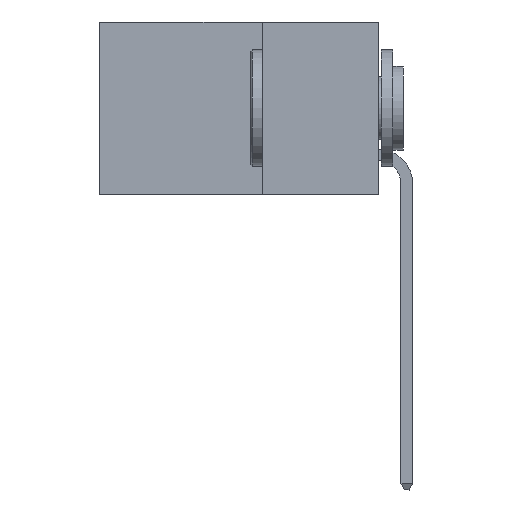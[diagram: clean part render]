
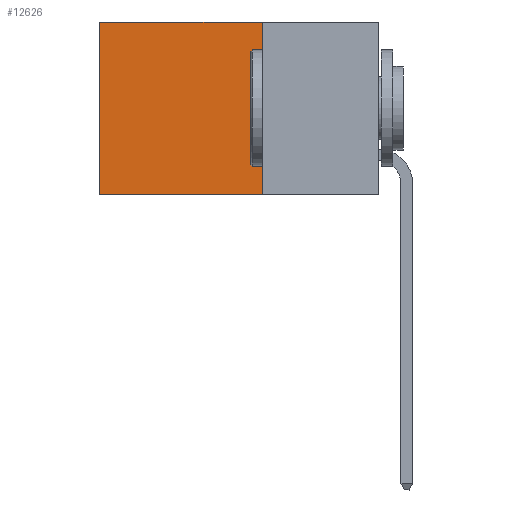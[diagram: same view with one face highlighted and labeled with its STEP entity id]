
A CAD part, left-side view. The second image highlights one B-rep face of the part: STEP entity #12626.
In plain terms, the highlighted planar face has unit normal (-1, 0, 0).
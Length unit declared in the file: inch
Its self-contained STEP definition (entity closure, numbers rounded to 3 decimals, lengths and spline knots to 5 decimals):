
#63 = CARTESIAN_POINT ( 'NONE',  ( 0.298, 0.25, -0.37 ) ) ;
#999 = PLANE ( 'NONE',  #11943 ) ;
#2259 = DIRECTION ( 'NONE',  ( 0., 0., -1. ) ) ;
#3012 = FACE_OUTER_BOUND ( 'NONE', #7542, .T. ) ;
#3633 = CARTESIAN_POINT ( 'NONE',  ( 0.298, 0.6, 0. ) ) ;
#3828 = DIRECTION ( 'NONE',  ( 0., 0., -1. ) ) ;
#4399 = VECTOR ( 'NONE', #9729, 39.37008 ) ;
#5087 = VECTOR ( 'NONE', #11997, 39.37008 ) ;
#5766 = VECTOR ( 'NONE', #6267, 39.37008 ) ;
#6267 = DIRECTION ( 'NONE',  ( 0., 1., 0. ) ) ;
#7542 = EDGE_LOOP ( 'NONE', ( #9388, #9931, #10273, #8222 ) ) ;
#7642 = VECTOR ( 'NONE', #3828, 39.37008 ) ;
#8222 = ORIENTED_EDGE ( 'NONE', *, *, #15827, .T. ) ;
#9388 = ORIENTED_EDGE ( 'NONE', *, *, #12764, .T. ) ;
#9648 = DIRECTION ( 'NONE',  ( 1., 0., 0. ) ) ;
#9729 = DIRECTION ( 'NONE',  ( 0., 0., -1. ) ) ;
#9931 = ORIENTED_EDGE ( 'NONE', *, *, #10472, .F. ) ;
#10273 = ORIENTED_EDGE ( 'NONE', *, *, #10363, .F. ) ;
#10280 = CARTESIAN_POINT ( 'NONE',  ( 0.298, 0.25, 0. ) ) ;
#10363 = EDGE_CURVE ( 'NONE', #15689, #11146, #13837, .T. ) ;
#10472 = EDGE_CURVE ( 'NONE', #11146, #15243, #15586, .T. ) ;
#10766 = CARTESIAN_POINT ( 'NONE',  ( 0.298, 0.25, 0. ) ) ;
#11146 = VERTEX_POINT ( 'NONE', #14893 ) ;
#11212 = CARTESIAN_POINT ( 'NONE',  ( 0.298, 0.6, 0. ) ) ;
#11943 = AXIS2_PLACEMENT_3D ( 'NONE', #15807, #9648, #2259 ) ;
#11997 = DIRECTION ( 'NONE',  ( 0., 1., 0. ) ) ;
#12626 = ADVANCED_FACE ( 'NONE', ( #3012 ), #999, .F. ) ;
#12764 = EDGE_CURVE ( 'NONE', #13867, #15243, #13815, .T. ) ;
#13139 = CARTESIAN_POINT ( 'NONE',  ( 0.298, 0.6, -0.37 ) ) ;
#13440 = CARTESIAN_POINT ( 'NONE',  ( 0.298, 0.25, 0. ) ) ;
#13815 = LINE ( 'NONE', #11212, #7642 ) ;
#13837 = LINE ( 'NONE', #13440, #4399 ) ;
#13867 = VERTEX_POINT ( 'NONE', #3633 ) ;
#14893 = CARTESIAN_POINT ( 'NONE',  ( 0.298, 0.25, -0.37 ) ) ;
#15243 = VERTEX_POINT ( 'NONE', #13139 ) ;
#15284 = LINE ( 'NONE', #10766, #5087 ) ;
#15586 = LINE ( 'NONE', #63, #5766 ) ;
#15689 = VERTEX_POINT ( 'NONE', #10280 ) ;
#15807 = CARTESIAN_POINT ( 'NONE',  ( 0.298, 0.25, 0. ) ) ;
#15827 = EDGE_CURVE ( 'NONE', #15689, #13867, #15284, .T. ) ;
